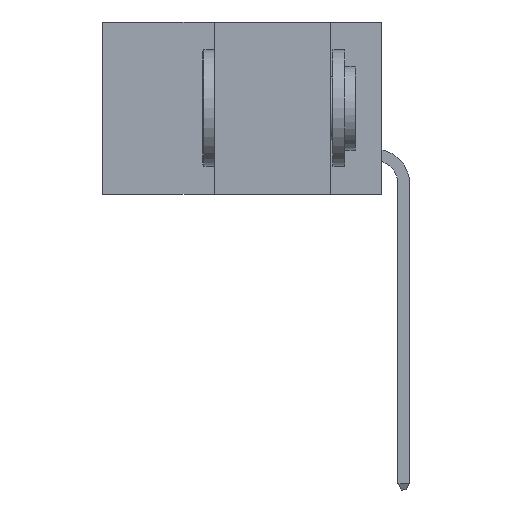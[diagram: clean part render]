
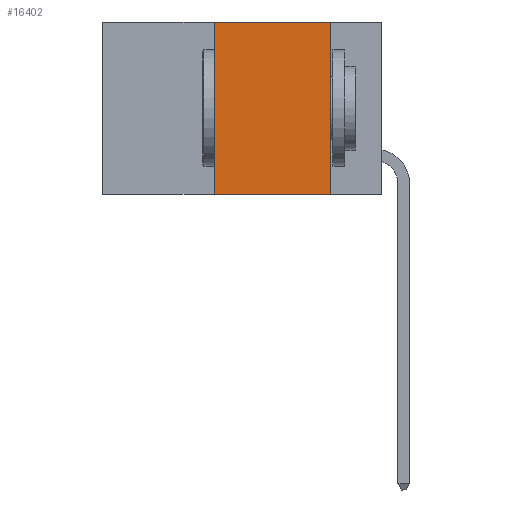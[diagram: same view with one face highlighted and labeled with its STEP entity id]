
A CAD part, left-side view. The second image highlights one B-rep face of the part: STEP entity #16402.
In plain terms, the highlighted planar face has unit normal (-1, 0, 0).
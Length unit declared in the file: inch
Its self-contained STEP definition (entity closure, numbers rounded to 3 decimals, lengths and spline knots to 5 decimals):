
#178 = DIRECTION ( 'NONE',  ( 0., 0., -1. ) ) ;
#398 = CARTESIAN_POINT ( 'NONE',  ( 0., 0.6, -0.37 ) ) ;
#1416 = CARTESIAN_POINT ( 'NONE',  ( 0., 0.11, 0. ) ) ;
#1648 = VERTEX_POINT ( 'NONE', #10610 ) ;
#3566 = EDGE_CURVE ( 'NONE', #10341, #16270, #13526, .T. ) ;
#4166 = ORIENTED_EDGE ( 'NONE', *, *, #19381, .T. ) ;
#5034 = VECTOR ( 'NONE', #15554, 39.37008 ) ;
#5111 = DIRECTION ( 'NONE',  ( 1., 0., 0. ) ) ;
#5168 = ORIENTED_EDGE ( 'NONE', *, *, #18363, .F. ) ;
#6103 = CARTESIAN_POINT ( 'NONE',  ( 0., 0.36, 0. ) ) ;
#6196 = FACE_OUTER_BOUND ( 'NONE', #10874, .T. ) ;
#6356 = VECTOR ( 'NONE', #15577, 39.37008 ) ;
#6960 = DIRECTION ( 'NONE',  ( 0., -1., 0. ) ) ;
#8977 = CARTESIAN_POINT ( 'NONE',  ( 0., 0.11, -0.37 ) ) ;
#8994 = LINE ( 'NONE', #13187, #9487 ) ;
#9158 = ORIENTED_EDGE ( 'NONE', *, *, #15211, .F. ) ;
#9487 = VECTOR ( 'NONE', #178, 39.37008 ) ;
#9867 = CARTESIAN_POINT ( 'NONE',  ( 0., 0.6, 0. ) ) ;
#10341 = VERTEX_POINT ( 'NONE', #12126 ) ;
#10582 = LINE ( 'NONE', #6103, #6356 ) ;
#10610 = CARTESIAN_POINT ( 'NONE',  ( 0., 0.36, -0.37 ) ) ;
#10874 = EDGE_LOOP ( 'NONE', ( #9158, #13877, #5168, #4166 ) ) ;
#12126 = CARTESIAN_POINT ( 'NONE',  ( 0., 0.36, 0. ) ) ;
#13187 = CARTESIAN_POINT ( 'NONE',  ( 0., 0.11, 0. ) ) ;
#13526 = LINE ( 'NONE', #15722, #5034 ) ;
#13877 = ORIENTED_EDGE ( 'NONE', *, *, #3566, .F. ) ;
#14786 = VECTOR ( 'NONE', #6960, 39.37008 ) ;
#15211 = EDGE_CURVE ( 'NONE', #16270, #16051, #8994, .T. ) ;
#15554 = DIRECTION ( 'NONE',  ( 0., -1., 0. ) ) ;
#15577 = DIRECTION ( 'NONE',  ( 0., 0., 1. ) ) ;
#15722 = CARTESIAN_POINT ( 'NONE',  ( 0., 0.6, 0. ) ) ;
#16051 = VERTEX_POINT ( 'NONE', #8977 ) ;
#16171 = DIRECTION ( 'NONE',  ( 0., 0., -1. ) ) ;
#16270 = VERTEX_POINT ( 'NONE', #1416 ) ;
#16402 = ADVANCED_FACE ( 'NONE', ( #6196 ), #19264, .F. ) ;
#18363 = EDGE_CURVE ( 'NONE', #1648, #10341, #10582, .T. ) ;
#19264 = PLANE ( 'NONE',  #19864 ) ;
#19381 = EDGE_CURVE ( 'NONE', #1648, #16051, #19397, .T. ) ;
#19397 = LINE ( 'NONE', #398, #14786 ) ;
#19864 = AXIS2_PLACEMENT_3D ( 'NONE', #9867, #5111, #16171 ) ;
